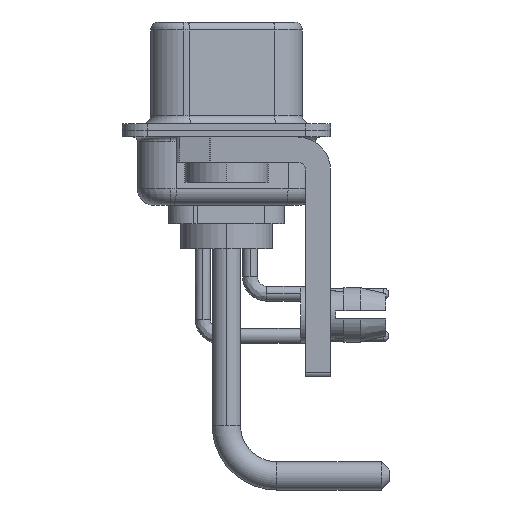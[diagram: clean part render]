
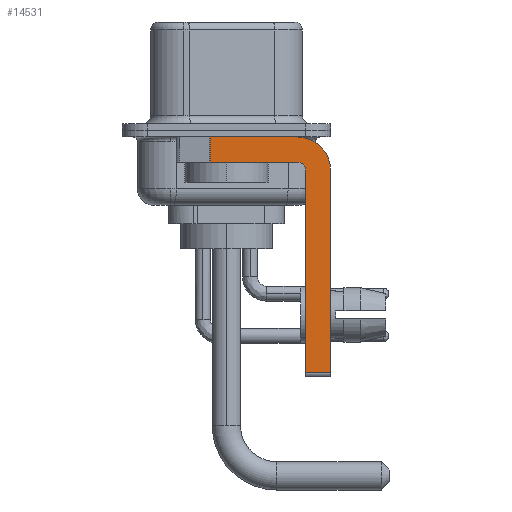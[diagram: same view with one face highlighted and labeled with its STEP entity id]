
A CAD part, left-side view. The second image highlights one B-rep face of the part: STEP entity #14531.
In plain terms, the highlighted planar face has unit normal (-1, 0, 0).
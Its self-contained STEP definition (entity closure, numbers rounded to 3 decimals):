
#12 = LINE ( 'NONE', #12742, #25988 ) ;
#981 = ORIENTED_EDGE ( 'NONE', *, *, #1259, .F. ) ;
#1259 = EDGE_CURVE ( 'NONE', #21428, #26963, #8272, .T. ) ;
#2504 = CARTESIAN_POINT ( 'NONE',  ( -2.9, -4.75, -14.55 ) ) ;
#3072 = ORIENTED_EDGE ( 'NONE', *, *, #4396, .T. ) ;
#3731 = DIRECTION ( 'NONE',  ( 0., 0., 1. ) ) ;
#3927 = LINE ( 'NONE', #6273, #5306 ) ;
#4396 = EDGE_CURVE ( 'NONE', #9459, #10288, #27056, .T. ) ;
#4734 = CARTESIAN_POINT ( 'NONE',  ( -2.9, -4.25, -1.9 ) ) ;
#4936 = AXIS2_PLACEMENT_3D ( 'NONE', #26612, #9904, #17893 ) ;
#5306 = VECTOR ( 'NONE', #6001, 1000. ) ;
#5706 = EDGE_CURVE ( 'NONE', #15223, #10288, #23496, .T. ) ;
#5809 = CARTESIAN_POINT ( 'NONE',  ( -2.9, -6.25, -2.4 ) ) ;
#6001 = DIRECTION ( 'NONE',  ( 0., 0., 1. ) ) ;
#6145 = ORIENTED_EDGE ( 'NONE', *, *, #5706, .F. ) ;
#6273 = CARTESIAN_POINT ( 'NONE',  ( -2.9, -4.75, -14.8 ) ) ;
#6721 = ORIENTED_EDGE ( 'NONE', *, *, #10693, .F. ) ;
#7021 = CARTESIAN_POINT ( 'NONE',  ( -2.9, -4.75, -2.4 ) ) ;
#8272 = LINE ( 'NONE', #5809, #14110 ) ;
#9424 = ORIENTED_EDGE ( 'NONE', *, *, #21785, .F. ) ;
#9459 = VERTEX_POINT ( 'NONE', #10089 ) ;
#9904 = DIRECTION ( 'NONE',  ( 1., 0., 0. ) ) ;
#10089 = CARTESIAN_POINT ( 'NONE',  ( -2.9, 0.978, -0.4 ) ) ;
#10288 = VERTEX_POINT ( 'NONE', #26845 ) ;
#10693 = EDGE_CURVE ( 'NONE', #14362, #24507, #3927, .T. ) ;
#11191 = DIRECTION ( 'NONE',  ( -1., 0., 0. ) ) ;
#11304 = EDGE_CURVE ( 'NONE', #9459, #15936, #12, .T. ) ;
#11528 = DIRECTION ( 'NONE',  ( 1., 0., 0. ) ) ;
#11926 = CARTESIAN_POINT ( 'NONE',  ( -2.9, -4.25, -2.4 ) ) ;
#12502 = EDGE_CURVE ( 'NONE', #14362, #26963, #19956, .T. ) ;
#12742 = CARTESIAN_POINT ( 'NONE',  ( -2.9, 3., -0.4 ) ) ;
#13675 = CARTESIAN_POINT ( 'NONE',  ( -2.9, -6.25, -14.55 ) ) ;
#14110 = VECTOR ( 'NONE', #16373, 1000. ) ;
#14362 = VERTEX_POINT ( 'NONE', #2504 ) ;
#14442 = CARTESIAN_POINT ( 'NONE',  ( -2.9, -4.25, -0.4 ) ) ;
#14531 = ADVANCED_FACE ( 'NONE', ( #20158 ), #19776, .F. ) ;
#14667 = DIRECTION ( 'NONE',  ( 0., -1., 0. ) ) ;
#14683 = VECTOR ( 'NONE', #22250, 1000. ) ;
#15223 = VERTEX_POINT ( 'NONE', #25296 ) ;
#15250 = VECTOR ( 'NONE', #21455, 1000. ) ;
#15654 = AXIS2_PLACEMENT_3D ( 'NONE', #11926, #11528, #22071 ) ;
#15936 = VERTEX_POINT ( 'NONE', #14442 ) ;
#16309 = CIRCLE ( 'NONE', #21114, 0.5 ) ;
#16373 = DIRECTION ( 'NONE',  ( 0., 0., -1. ) ) ;
#16386 = EDGE_LOOP ( 'NONE', ( #22587, #3072, #6145, #24606, #6721, #17707, #981, #9424 ) ) ;
#16670 = DIRECTION ( 'NONE',  ( 0., 0., -1. ) ) ;
#16768 = CIRCLE ( 'NONE', #4936, 2. ) ;
#17707 = ORIENTED_EDGE ( 'NONE', *, *, #12502, .T. ) ;
#17776 = VECTOR ( 'NONE', #16670, 1000. ) ;
#17893 = DIRECTION ( 'NONE',  ( 0., 0., -1. ) ) ;
#19776 = PLANE ( 'NONE',  #15654 ) ;
#19956 = LINE ( 'NONE', #26341, #14683 ) ;
#20158 = FACE_OUTER_BOUND ( 'NONE', #16386, .T. ) ;
#20912 = CARTESIAN_POINT ( 'NONE',  ( -2.9, 0.978, -1.9 ) ) ;
#21114 = AXIS2_PLACEMENT_3D ( 'NONE', #22497, #11191, #3731 ) ;
#21428 = VERTEX_POINT ( 'NONE', #27050 ) ;
#21455 = DIRECTION ( 'NONE',  ( 0., 1., 0. ) ) ;
#21785 = EDGE_CURVE ( 'NONE', #15936, #21428, #16768, .T. ) ;
#22071 = DIRECTION ( 'NONE',  ( 0., 0., -1. ) ) ;
#22250 = DIRECTION ( 'NONE',  ( 0., -1., 0. ) ) ;
#22497 = CARTESIAN_POINT ( 'NONE',  ( -2.9, -4.25, -2.4 ) ) ;
#22587 = ORIENTED_EDGE ( 'NONE', *, *, #11304, .F. ) ;
#23496 = LINE ( 'NONE', #4734, #15250 ) ;
#24219 = EDGE_CURVE ( 'NONE', #24507, #15223, #16309, .T. ) ;
#24507 = VERTEX_POINT ( 'NONE', #7021 ) ;
#24606 = ORIENTED_EDGE ( 'NONE', *, *, #24219, .F. ) ;
#25296 = CARTESIAN_POINT ( 'NONE',  ( -2.9, -4.25, -1.9 ) ) ;
#25988 = VECTOR ( 'NONE', #14667, 1000. ) ;
#26341 = CARTESIAN_POINT ( 'NONE',  ( -2.9, -4.25, -14.55 ) ) ;
#26612 = CARTESIAN_POINT ( 'NONE',  ( -2.9, -4.25, -2.4 ) ) ;
#26845 = CARTESIAN_POINT ( 'NONE',  ( -2.9, 0.978, -1.9 ) ) ;
#26963 = VERTEX_POINT ( 'NONE', #13675 ) ;
#27050 = CARTESIAN_POINT ( 'NONE',  ( -2.9, -6.25, -2.4 ) ) ;
#27056 = LINE ( 'NONE', #20912, #17776 ) ;
